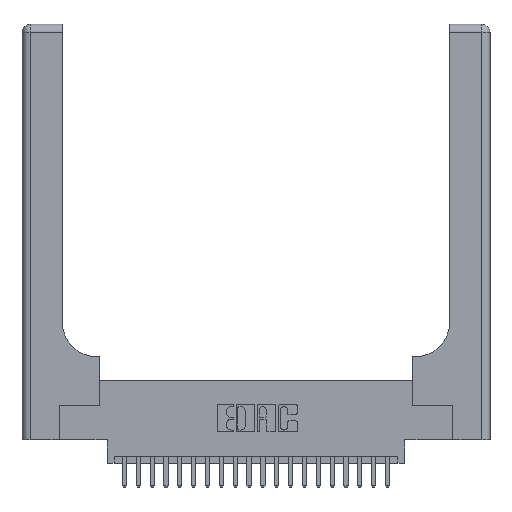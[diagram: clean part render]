
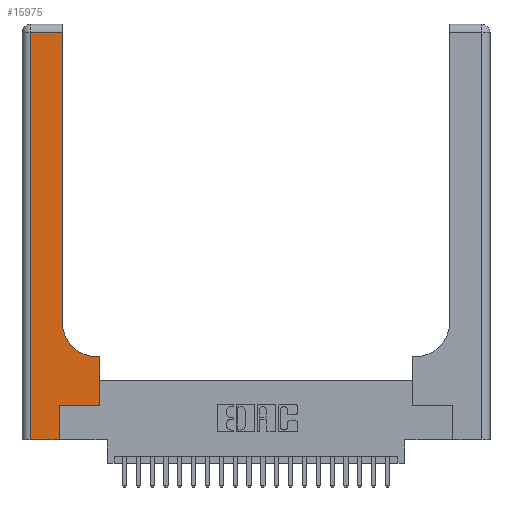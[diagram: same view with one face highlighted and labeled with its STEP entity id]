
A CAD part, top view. The second image highlights one B-rep face of the part: STEP entity #15975.
In plain terms, the highlighted planar face has unit normal (0, 0, 1).
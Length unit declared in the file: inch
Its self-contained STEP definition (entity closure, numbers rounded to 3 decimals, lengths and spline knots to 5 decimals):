
#575 = LINE ( 'NONE', #3925, #6957 ) ;
#580 = CARTESIAN_POINT ( 'NONE',  ( 0., 2.94, 0.37 ) ) ;
#1106 = VECTOR ( 'NONE', #21478, 39.37008 ) ;
#1273 = DIRECTION ( 'NONE',  ( 0., 1., 0. ) ) ;
#1881 = CARTESIAN_POINT ( 'NONE',  ( 0.06, 0., 0.37 ) ) ;
#1951 = ORIENTED_EDGE ( 'NONE', *, *, #10656, .T. ) ;
#2087 = VERTEX_POINT ( 'NONE', #22998 ) ;
#3016 = CARTESIAN_POINT ( 'NONE',  ( 0.5585, 0.25, 0.37 ) ) ;
#3250 = DIRECTION ( 'NONE',  ( 1., 0., 0. ) ) ;
#3925 = CARTESIAN_POINT ( 'NONE',  ( 0.2915, 3., 0.37 ) ) ;
#3938 = VECTOR ( 'NONE', #16397, 39.37008 ) ;
#4193 = ORIENTED_EDGE ( 'NONE', *, *, #5443, .T. ) ;
#4804 = ORIENTED_EDGE ( 'NONE', *, *, #23531, .T. ) ;
#4932 = CARTESIAN_POINT ( 'NONE',  ( 0.5415, 0.85, 0.37 ) ) ;
#5443 = EDGE_CURVE ( 'NONE', #22735, #15690, #13697, .T. ) ;
#5656 = VERTEX_POINT ( 'NONE', #20916 ) ;
#5697 = DIRECTION ( 'NONE',  ( 0., -1., 0. ) ) ;
#6057 = EDGE_CURVE ( 'NONE', #23223, #12545, #8963, .T. ) ;
#6119 = CARTESIAN_POINT ( 'NONE',  ( 0., 3., 0.37 ) ) ;
#6957 = VECTOR ( 'NONE', #7634, 39.37008 ) ;
#7244 = CARTESIAN_POINT ( 'NONE',  ( 0.269, 0.25, 0.37 ) ) ;
#7634 = DIRECTION ( 'NONE',  ( 0., 1., 0. ) ) ;
#8205 = DIRECTION ( 'NONE',  ( -1., 0., 0. ) ) ;
#8755 = VECTOR ( 'NONE', #8205, 39.37008 ) ;
#8963 = LINE ( 'NONE', #3016, #1106 ) ;
#9672 = LINE ( 'NONE', #23591, #20156 ) ;
#9689 = AXIS2_PLACEMENT_3D ( 'NONE', #6119, #20947, #17300 ) ;
#9918 = VERTEX_POINT ( 'NONE', #22931 ) ;
#10084 = EDGE_CURVE ( 'NONE', #9918, #2087, #13724, .T. ) ;
#10381 = DIRECTION ( 'NONE',  ( 1., 0., 0. ) ) ;
#10437 = CARTESIAN_POINT ( 'NONE',  ( 0.2915, 2.94, 0.37 ) ) ;
#10498 = LINE ( 'NONE', #23557, #20095 ) ;
#10656 = EDGE_CURVE ( 'NONE', #5656, #15174, #10498, .T. ) ;
#10966 = VECTOR ( 'NONE', #5697, 39.37008 ) ;
#11120 = EDGE_CURVE ( 'NONE', #2087, #22735, #575, .T. ) ;
#11134 = ORIENTED_EDGE ( 'NONE', *, *, #6057, .T. ) ;
#11469 = FACE_OUTER_BOUND ( 'NONE', #13194, .T. ) ;
#12545 = VERTEX_POINT ( 'NONE', #12635 ) ;
#12635 = CARTESIAN_POINT ( 'NONE',  ( 0.5585, 0.6, 0.37 ) ) ;
#12807 = CARTESIAN_POINT ( 'NONE',  ( 0.2915, 0.6, 0.37 ) ) ;
#13194 = EDGE_LOOP ( 'NONE', ( #17745, #4193, #13296, #18626, #1951, #4804, #11134, #14395, #20764 ) ) ;
#13296 = ORIENTED_EDGE ( 'NONE', *, *, #19909, .T. ) ;
#13420 = CARTESIAN_POINT ( 'NONE',  ( 0.269, 0.25, 0.37 ) ) ;
#13697 = LINE ( 'NONE', #580, #8755 ) ;
#13724 = CIRCLE ( 'NONE', #20851, 0.25 ) ;
#14053 = DIRECTION ( 'NONE',  ( 0., 0., -1. ) ) ;
#14395 = ORIENTED_EDGE ( 'NONE', *, *, #21602, .T. ) ;
#14929 = CARTESIAN_POINT ( 'NONE',  ( 0.06, 3., 0.37 ) ) ;
#15174 = VERTEX_POINT ( 'NONE', #7244 ) ;
#15264 = PLANE ( 'NONE',  #9689 ) ;
#15690 = VERTEX_POINT ( 'NONE', #20223 ) ;
#15975 = ADVANCED_FACE ( 'NONE', ( #11469 ), #15264, .F. ) ;
#16397 = DIRECTION ( 'NONE',  ( -1., 0., 0. ) ) ;
#16471 = CARTESIAN_POINT ( 'NONE',  ( 0.5585, 0.25, 0.37 ) ) ;
#16928 = EDGE_CURVE ( 'NONE', #18793, #5656, #9672, .T. ) ;
#17036 = LINE ( 'NONE', #12807, #3938 ) ;
#17300 = DIRECTION ( 'NONE',  ( -1., 0., 0. ) ) ;
#17745 = ORIENTED_EDGE ( 'NONE', *, *, #11120, .T. ) ;
#18626 = ORIENTED_EDGE ( 'NONE', *, *, #16928, .T. ) ;
#18793 = VERTEX_POINT ( 'NONE', #1881 ) ;
#19909 = EDGE_CURVE ( 'NONE', #15690, #18793, #20825, .T. ) ;
#20095 = VECTOR ( 'NONE', #1273, 39.37008 ) ;
#20156 = VECTOR ( 'NONE', #10381, 39.37008 ) ;
#20223 = CARTESIAN_POINT ( 'NONE',  ( 0.06, 2.94, 0.37 ) ) ;
#20692 = LINE ( 'NONE', #13420, #22197 ) ;
#20764 = ORIENTED_EDGE ( 'NONE', *, *, #10084, .T. ) ;
#20825 = LINE ( 'NONE', #14929, #10966 ) ;
#20851 = AXIS2_PLACEMENT_3D ( 'NONE', #4932, #14053, #3250 ) ;
#20916 = CARTESIAN_POINT ( 'NONE',  ( 0.269, 0., 0.37 ) ) ;
#20947 = DIRECTION ( 'NONE',  ( 0., 0., -1. ) ) ;
#21478 = DIRECTION ( 'NONE',  ( 0., 1., 0. ) ) ;
#21602 = EDGE_CURVE ( 'NONE', #12545, #9918, #17036, .T. ) ;
#22197 = VECTOR ( 'NONE', #22471, 39.37008 ) ;
#22471 = DIRECTION ( 'NONE',  ( 1., 0., 0. ) ) ;
#22735 = VERTEX_POINT ( 'NONE', #10437 ) ;
#22931 = CARTESIAN_POINT ( 'NONE',  ( 0.5415, 0.6, 0.37 ) ) ;
#22998 = CARTESIAN_POINT ( 'NONE',  ( 0.2915, 0.85, 0.37 ) ) ;
#23223 = VERTEX_POINT ( 'NONE', #16471 ) ;
#23531 = EDGE_CURVE ( 'NONE', #15174, #23223, #20692, .T. ) ;
#23557 = CARTESIAN_POINT ( 'NONE',  ( 0.269, 0., 0.37 ) ) ;
#23591 = CARTESIAN_POINT ( 'NONE',  ( 0., 0., 0.37 ) ) ;
